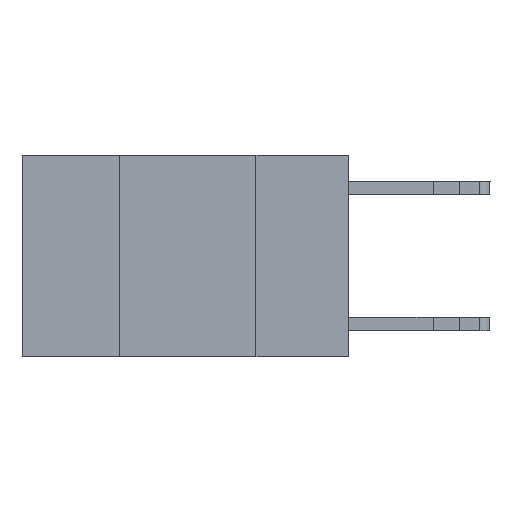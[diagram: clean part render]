
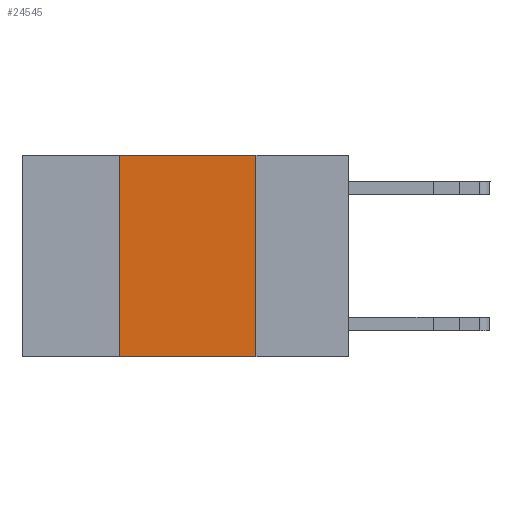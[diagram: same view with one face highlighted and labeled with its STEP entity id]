
A CAD part, left-side view. The second image highlights one B-rep face of the part: STEP entity #24545.
In plain terms, the highlighted planar face has unit normal (-1, 0, 0).
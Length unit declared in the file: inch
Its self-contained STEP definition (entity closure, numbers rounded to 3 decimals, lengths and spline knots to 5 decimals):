
#144 = ORIENTED_EDGE ( 'NONE', *, *, #26781, .F. ) ;
#270 = CARTESIAN_POINT ( 'NONE',  ( 0., 0.6, 0. ) ) ;
#787 = CARTESIAN_POINT ( 'NONE',  ( 0., 0.17, -0.37 ) ) ;
#1838 = VECTOR ( 'NONE', #17199, 39.37008 ) ;
#3319 = VERTEX_POINT ( 'NONE', #10546 ) ;
#3888 = DIRECTION ( 'NONE',  ( 0., 0., 1. ) ) ;
#4158 = LINE ( 'NONE', #12492, #10032 ) ;
#6502 = LINE ( 'NONE', #27305, #1838 ) ;
#6650 = DIRECTION ( 'NONE',  ( 0., -1., 0. ) ) ;
#6658 = FACE_OUTER_BOUND ( 'NONE', #11063, .T. ) ;
#6686 = VERTEX_POINT ( 'NONE', #787 ) ;
#6775 = LINE ( 'NONE', #7193, #20542 ) ;
#7063 = PLANE ( 'NONE',  #15611 ) ;
#7193 = CARTESIAN_POINT ( 'NONE',  ( 0., 0.6, -0.37 ) ) ;
#8126 = CARTESIAN_POINT ( 'NONE',  ( 0., 0.6, 0. ) ) ;
#8178 = EDGE_CURVE ( 'NONE', #3319, #22217, #4158, .T. ) ;
#8742 = DIRECTION ( 'NONE',  ( 0., 0., -1. ) ) ;
#9688 = EDGE_CURVE ( 'NONE', #3319, #6686, #6775, .T. ) ;
#10032 = VECTOR ( 'NONE', #3888, 39.37008 ) ;
#10342 = DIRECTION ( 'NONE',  ( 0., -1., 0. ) ) ;
#10546 = CARTESIAN_POINT ( 'NONE',  ( 0., 0.42, -0.37 ) ) ;
#10593 = ORIENTED_EDGE ( 'NONE', *, *, #9688, .T. ) ;
#11063 = EDGE_LOOP ( 'NONE', ( #11368, #144, #16160, #10593 ) ) ;
#11368 = ORIENTED_EDGE ( 'NONE', *, *, #24308, .F. ) ;
#12492 = CARTESIAN_POINT ( 'NONE',  ( 0., 0.42, 0. ) ) ;
#15144 = DIRECTION ( 'NONE',  ( 1., 0., 0. ) ) ;
#15611 = AXIS2_PLACEMENT_3D ( 'NONE', #270, #15144, #8742 ) ;
#16160 = ORIENTED_EDGE ( 'NONE', *, *, #8178, .F. ) ;
#17000 = VECTOR ( 'NONE', #10342, 39.37008 ) ;
#17199 = DIRECTION ( 'NONE',  ( 0., 0., -1. ) ) ;
#18925 = CARTESIAN_POINT ( 'NONE',  ( 0., 0.42, 0. ) ) ;
#20542 = VECTOR ( 'NONE', #6650, 39.37008 ) ;
#22217 = VERTEX_POINT ( 'NONE', #18925 ) ;
#24308 = EDGE_CURVE ( 'NONE', #26710, #6686, #6502, .T. ) ;
#24545 = ADVANCED_FACE ( 'NONE', ( #6658 ), #7063, .F. ) ;
#24921 = CARTESIAN_POINT ( 'NONE',  ( 0., 0.17, 0. ) ) ;
#26710 = VERTEX_POINT ( 'NONE', #24921 ) ;
#26781 = EDGE_CURVE ( 'NONE', #22217, #26710, #27123, .T. ) ;
#27123 = LINE ( 'NONE', #8126, #17000 ) ;
#27305 = CARTESIAN_POINT ( 'NONE',  ( 0., 0.17, 0. ) ) ;
